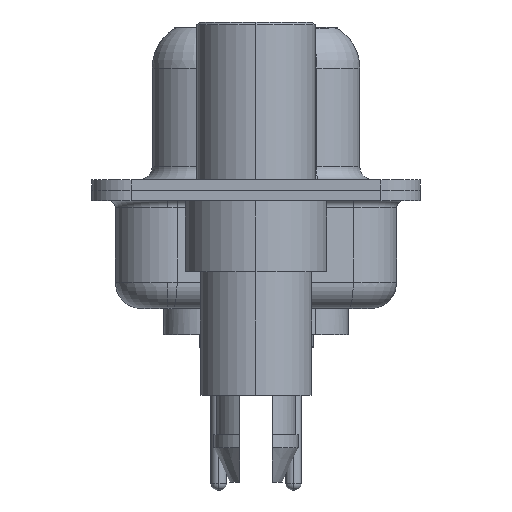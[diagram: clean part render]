
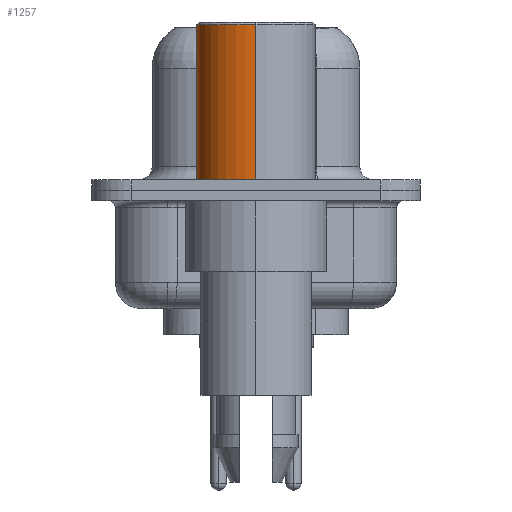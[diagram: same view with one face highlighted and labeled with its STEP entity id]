
A CAD part, left-side view. The second image highlights one B-rep face of the part: STEP entity #1257.
In plain terms, the highlighted cylindrical face has radius 2.25 mm (diameter 4.5 mm), a partial arc.
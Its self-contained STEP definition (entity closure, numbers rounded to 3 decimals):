
#1257 = ADVANCED_FACE ( 'NONE', ( #15035 ), #16821, .T. ) ;
#1365 = CARTESIAN_POINT ( 'NONE',  ( 2.25, 0., 0.4 ) ) ;
#2154 = CARTESIAN_POINT ( 'NONE',  ( 0., 0., 6.3 ) ) ;
#2261 = DIRECTION ( 'NONE',  ( 0., 0., 1. ) ) ;
#2372 = CARTESIAN_POINT ( 'NONE',  ( 2.25, 0., 6.3 ) ) ;
#2524 = LINE ( 'NONE', #17223, #13014 ) ;
#2575 = CARTESIAN_POINT ( 'NONE',  ( -2.25, 0., 0.581 ) ) ;
#3602 = ORIENTED_EDGE ( 'NONE', *, *, #7399, .F. ) ;
#3899 = VERTEX_POINT ( 'NONE', #2372 ) ;
#4429 = DIRECTION ( 'NONE',  ( 1., 0., 0. ) ) ;
#5130 = LINE ( 'NONE', #2575, #13264 ) ;
#5830 = CIRCLE ( 'NONE', #12366, 2.25 ) ;
#6755 = DIRECTION ( 'NONE',  ( 1., 0., 0. ) ) ;
#7399 = EDGE_CURVE ( 'NONE', #3899, #18377, #5830, .T. ) ;
#7933 = CARTESIAN_POINT ( 'NONE',  ( -2.25, 0., 6.3 ) ) ;
#8193 = CARTESIAN_POINT ( 'NONE',  ( -2.25, 0., 0.4 ) ) ;
#9185 = EDGE_CURVE ( 'NONE', #25063, #18377, #5130, .T. ) ;
#10832 = VERTEX_POINT ( 'NONE', #1365 ) ;
#12366 = AXIS2_PLACEMENT_3D ( 'NONE', #2154, #23283, #6755 ) ;
#12440 = ORIENTED_EDGE ( 'NONE', *, *, #21409, .F. ) ;
#13014 = VECTOR ( 'NONE', #25588, 1000. ) ;
#13264 = VECTOR ( 'NONE', #23460, 1000. ) ;
#14051 = CARTESIAN_POINT ( 'NONE',  ( 0., 0., 0.4 ) ) ;
#14788 = ORIENTED_EDGE ( 'NONE', *, *, #9185, .T. ) ;
#15035 = FACE_OUTER_BOUND ( 'NONE', #26794, .T. ) ;
#16821 = CYLINDRICAL_SURFACE ( 'NONE', #21944, 2.25 ) ;
#17223 = CARTESIAN_POINT ( 'NONE',  ( 2.25, 0., 0.581 ) ) ;
#18027 = DIRECTION ( 'NONE',  ( 0., 0., 1. ) ) ;
#18377 = VERTEX_POINT ( 'NONE', #7933 ) ;
#18476 = EDGE_CURVE ( 'NONE', #10832, #25063, #21621, .T. ) ;
#18589 = ORIENTED_EDGE ( 'NONE', *, *, #18476, .T. ) ;
#19056 = CARTESIAN_POINT ( 'NONE',  ( 0., 0., 0.581 ) ) ;
#21409 = EDGE_CURVE ( 'NONE', #10832, #3899, #2524, .T. ) ;
#21621 = CIRCLE ( 'NONE', #25960, 2.25 ) ;
#21944 = AXIS2_PLACEMENT_3D ( 'NONE', #19056, #2261, #4429 ) ;
#23283 = DIRECTION ( 'NONE',  ( 0., 0., 1. ) ) ;
#23460 = DIRECTION ( 'NONE',  ( 0., 0., 1. ) ) ;
#24459 = DIRECTION ( 'NONE',  ( 1., 0., 0. ) ) ;
#25063 = VERTEX_POINT ( 'NONE', #8193 ) ;
#25588 = DIRECTION ( 'NONE',  ( 0., 0., 1. ) ) ;
#25960 = AXIS2_PLACEMENT_3D ( 'NONE', #14051, #18027, #24459 ) ;
#26794 = EDGE_LOOP ( 'NONE', ( #18589, #14788, #3602, #12440 ) ) ;
